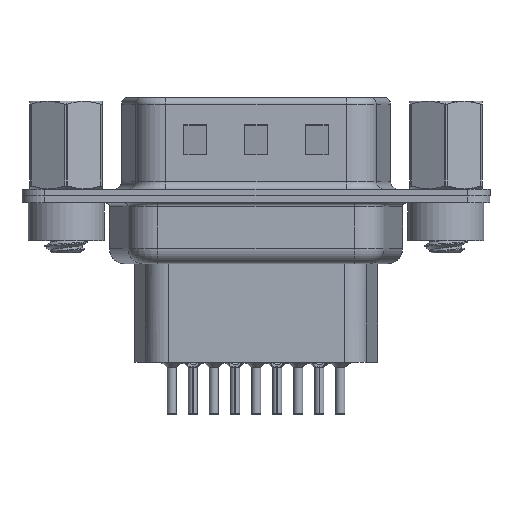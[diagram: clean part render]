
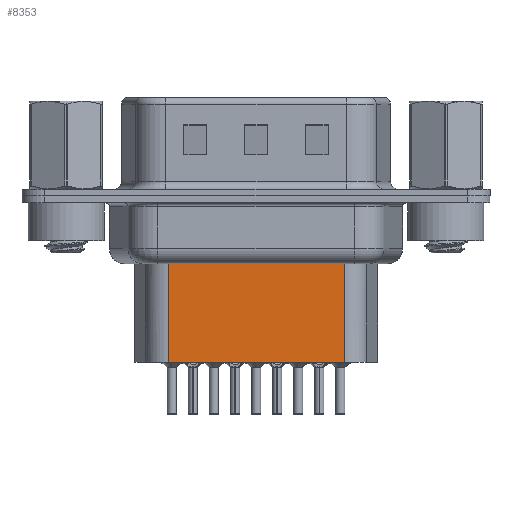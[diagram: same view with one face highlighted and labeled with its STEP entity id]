
A CAD part, front view. The second image highlights one B-rep face of the part: STEP entity #8353.
In plain terms, the highlighted planar face has unit normal (0, -1, 0).
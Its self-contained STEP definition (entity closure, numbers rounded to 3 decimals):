
#841 = VERTEX_POINT ( 'NONE', #11051 ) ;
#1433 = AXIS2_PLACEMENT_3D ( 'NONE', #16113, #16349, #21300 ) ;
#1441 = CARTESIAN_POINT ( 'NONE',  ( 18.294, -3.5, -4.097 ) ) ;
#2791 = EDGE_CURVE ( 'NONE', #17715, #841, #21007, .T. ) ;
#2954 = LINE ( 'NONE', #11945, #19534 ) ;
#3224 = ORIENTED_EDGE ( 'NONE', *, *, #7763, .F. ) ;
#3899 = VECTOR ( 'NONE', #8692, 1000. ) ;
#4627 = DIRECTION ( 'NONE',  ( -1., 0., 0. ) ) ;
#4847 = CARTESIAN_POINT ( 'NONE',  ( 18.294, -3.5, -3.1 ) ) ;
#5073 = DIRECTION ( 'NONE',  ( 0., 0., -1. ) ) ;
#7030 = CARTESIAN_POINT ( 'NONE',  ( 6.706, -3.5, -4.097 ) ) ;
#7327 = VECTOR ( 'NONE', #17169, 1000. ) ;
#7763 = EDGE_CURVE ( 'NONE', #841, #11438, #2954, .T. ) ;
#8236 = CARTESIAN_POINT ( 'NONE',  ( 6.459, -3.5, -4.097 ) ) ;
#8308 = CARTESIAN_POINT ( 'NONE',  ( 6.706, -3.5, -3.1 ) ) ;
#8353 = ADVANCED_FACE ( 'NONE', ( #12455 ), #9028, .T. ) ;
#8692 = DIRECTION ( 'NONE',  ( -1., 0., 0. ) ) ;
#9028 = PLANE ( 'NONE',  #1433 ) ;
#11051 = CARTESIAN_POINT ( 'NONE',  ( 18.294, -3.5, -10.95 ) ) ;
#11279 = VECTOR ( 'NONE', #5073, 1000. ) ;
#11438 = VERTEX_POINT ( 'NONE', #20713 ) ;
#11551 = EDGE_LOOP ( 'NONE', ( #16109, #17601, #12393, #3224 ) ) ;
#11945 = CARTESIAN_POINT ( 'NONE',  ( 6.706, -3.5, -10.95 ) ) ;
#12237 = LINE ( 'NONE', #8236, #3899 ) ;
#12393 = ORIENTED_EDGE ( 'NONE', *, *, #21783, .T. ) ;
#12455 = FACE_OUTER_BOUND ( 'NONE', #11551, .T. ) ;
#14171 = VERTEX_POINT ( 'NONE', #7030 ) ;
#16109 = ORIENTED_EDGE ( 'NONE', *, *, #2791, .F. ) ;
#16113 = CARTESIAN_POINT ( 'NONE',  ( 6.706, -3.5, -3.1 ) ) ;
#16349 = DIRECTION ( 'NONE',  ( 0., -1., 0. ) ) ;
#17169 = DIRECTION ( 'NONE',  ( 0., 0., -1. ) ) ;
#17195 = EDGE_CURVE ( 'NONE', #17715, #14171, #12237, .T. ) ;
#17601 = ORIENTED_EDGE ( 'NONE', *, *, #17195, .T. ) ;
#17715 = VERTEX_POINT ( 'NONE', #1441 ) ;
#19534 = VECTOR ( 'NONE', #4627, 1000. ) ;
#20713 = CARTESIAN_POINT ( 'NONE',  ( 6.706, -3.5, -10.95 ) ) ;
#21007 = LINE ( 'NONE', #4847, #11279 ) ;
#21300 = DIRECTION ( 'NONE',  ( 1., 0., 0. ) ) ;
#21783 = EDGE_CURVE ( 'NONE', #14171, #11438, #22828, .T. ) ;
#22828 = LINE ( 'NONE', #8308, #7327 ) ;
